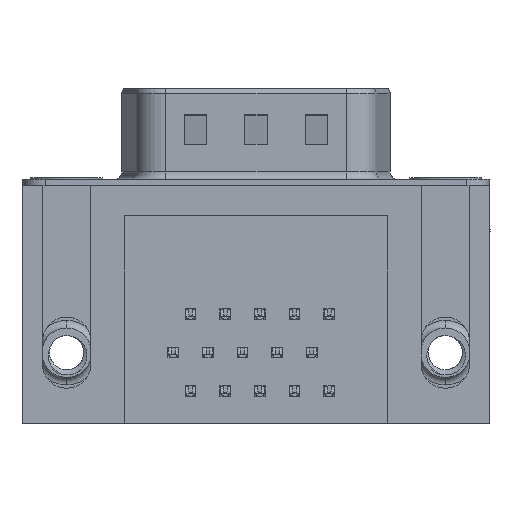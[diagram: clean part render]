
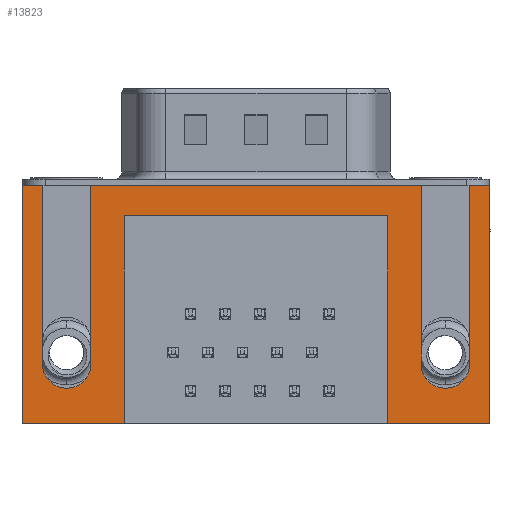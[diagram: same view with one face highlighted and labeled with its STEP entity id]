
A CAD part, front view. The second image highlights one B-rep face of the part: STEP entity #13823.
In plain terms, the highlighted planar face has unit normal (0, -1, 0).
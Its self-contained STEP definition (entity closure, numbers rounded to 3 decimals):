
#106 = DIRECTION ( 'NONE',  ( 0., 0., 1. ) ) ;
#407 = DIRECTION ( 'NONE',  ( 0., -1., 0. ) ) ;
#467 = ORIENTED_EDGE ( 'NONE', *, *, #11216, .F. ) ;
#515 = DIRECTION ( 'NONE',  ( 1., 0., 0. ) ) ;
#764 = VERTEX_POINT ( 'NONE', #19574 ) ;
#930 = CARTESIAN_POINT ( 'NONE',  ( -1.6, -6.275, 0. ) ) ;
#1017 = CARTESIAN_POINT ( 'NONE',  ( 26.59, -6.275, 0. ) ) ;
#1117 = CARTESIAN_POINT ( 'NONE',  ( -2.91, -6.275, -2.5 ) ) ;
#1310 = CARTESIAN_POINT ( 'NONE',  ( 23.39, -6.275, -11.78 ) ) ;
#1505 = EDGE_CURVE ( 'NONE', #8039, #16333, #14740, .T. ) ;
#1553 = VECTOR ( 'NONE', #17499, 1000. ) ;
#1867 = AXIS2_PLACEMENT_3D ( 'NONE', #20007, #10020, #106 ) ;
#1883 = LINE ( 'NONE', #6832, #10170 ) ;
#1933 = EDGE_CURVE ( 'NONE', #10922, #8039, #16270, .T. ) ;
#2094 = CARTESIAN_POINT ( 'NONE',  ( 26.59, -6.275, 0. ) ) ;
#2270 = ORIENTED_EDGE ( 'NONE', *, *, #19438, .F. ) ;
#2291 = DIRECTION ( 'NONE',  ( 0., 0., 1. ) ) ;
#2579 = VECTOR ( 'NONE', #10424, 1000. ) ;
#2657 = DIRECTION ( 'NONE',  ( 0., 0., -1. ) ) ;
#2797 = ORIENTED_EDGE ( 'NONE', *, *, #4100, .F. ) ;
#2808 = FACE_OUTER_BOUND ( 'NONE', #17017, .T. ) ;
#2905 = CARTESIAN_POINT ( 'NONE',  ( 27.9, -6.275, -2.5 ) ) ;
#2934 = VERTEX_POINT ( 'NONE', #20916 ) ;
#3137 = LINE ( 'NONE', #3846, #11400 ) ;
#3655 = LINE ( 'NONE', #18631, #11928 ) ;
#3657 = DIRECTION ( 'NONE',  ( 0., 0., 1. ) ) ;
#3846 = CARTESIAN_POINT ( 'NONE',  ( -2.91, -6.275, 0. ) ) ;
#3973 = CARTESIAN_POINT ( 'NONE',  ( 3.79, -6.275, -2. ) ) ;
#4032 = EDGE_CURVE ( 'NONE', #13349, #19043, #15791, .T. ) ;
#4100 = EDGE_CURVE ( 'NONE', #18681, #9261, #14753, .T. ) ;
#4137 = DIRECTION ( 'NONE',  ( -1., 0., 0. ) ) ;
#4527 = CARTESIAN_POINT ( 'NONE',  ( 23.39, -6.275, 0. ) ) ;
#4547 = EDGE_CURVE ( 'NONE', #9043, #7284, #19715, .T. ) ;
#4594 = CARTESIAN_POINT ( 'NONE',  ( 27.9, -6.275, 0. ) ) ;
#4648 = CARTESIAN_POINT ( 'NONE',  ( 1.6, -6.275, -11.78 ) ) ;
#4765 = VERTEX_POINT ( 'NONE', #12665 ) ;
#4778 = ORIENTED_EDGE ( 'NONE', *, *, #17791, .F. ) ;
#4785 = CARTESIAN_POINT ( 'NONE',  ( 27.9, -6.275, -15.7 ) ) ;
#5122 = CARTESIAN_POINT ( 'NONE',  ( -2.91, -6.275, 0. ) ) ;
#5206 = VECTOR ( 'NONE', #14465, 1000. ) ;
#5345 = VERTEX_POINT ( 'NONE', #4785 ) ;
#5378 = AXIS2_PLACEMENT_3D ( 'NONE', #10319, #407, #11957 ) ;
#5626 = ORIENTED_EDGE ( 'NONE', *, *, #19762, .F. ) ;
#5706 = AXIS2_PLACEMENT_3D ( 'NONE', #1117, #17706, #7795 ) ;
#5830 = CARTESIAN_POINT ( 'NONE',  ( 3.79, -6.275, -2. ) ) ;
#5968 = VECTOR ( 'NONE', #15062, 1000. ) ;
#6076 = CARTESIAN_POINT ( 'NONE',  ( 21.2, -6.275, -2. ) ) ;
#6199 = DIRECTION ( 'NONE',  ( 0., 0., -1. ) ) ;
#6203 = EDGE_CURVE ( 'NONE', #7284, #20278, #16646, .T. ) ;
#6571 = VECTOR ( 'NONE', #2657, 1000. ) ;
#6599 = DIRECTION ( 'NONE',  ( 0., 0., -1. ) ) ;
#6826 = DIRECTION ( 'NONE',  ( 1., 0., 0. ) ) ;
#6832 = CARTESIAN_POINT ( 'NONE',  ( -2.91, -6.275, 0. ) ) ;
#7178 = CARTESIAN_POINT ( 'NONE',  ( -2.91, -6.275, -2.5 ) ) ;
#7284 = VERTEX_POINT ( 'NONE', #6076 ) ;
#7589 = VECTOR ( 'NONE', #6826, 1000. ) ;
#7609 = CARTESIAN_POINT ( 'NONE',  ( 27.9, -6.275, -15.7 ) ) ;
#7769 = ORIENTED_EDGE ( 'NONE', *, *, #4032, .F. ) ;
#7795 = DIRECTION ( 'NONE',  ( 0., 0., -1. ) ) ;
#7887 = CARTESIAN_POINT ( 'NONE',  ( -1.6, -6.275, 0. ) ) ;
#8039 = VERTEX_POINT ( 'NONE', #4648 ) ;
#8467 = DIRECTION ( 'NONE',  ( 1., 0., 0. ) ) ;
#8896 = ORIENTED_EDGE ( 'NONE', *, *, #4547, .F. ) ;
#9043 = VERTEX_POINT ( 'NONE', #17432 ) ;
#9144 = AXIS2_PLACEMENT_3D ( 'NONE', #12203, #15199, #14990 ) ;
#9261 = VERTEX_POINT ( 'NONE', #17936 ) ;
#9319 = ORIENTED_EDGE ( 'NONE', *, *, #20046, .F. ) ;
#9422 = CARTESIAN_POINT ( 'NONE',  ( 0., -6.275, -11.78 ) ) ;
#9679 = EDGE_CURVE ( 'NONE', #4765, #12709, #16786, .T. ) ;
#9837 = CARTESIAN_POINT ( 'NONE',  ( 1.6, -6.275, 0. ) ) ;
#10020 = DIRECTION ( 'NONE',  ( 0., -1., 0. ) ) ;
#10170 = VECTOR ( 'NONE', #8467, 1000. ) ;
#10319 = CARTESIAN_POINT ( 'NONE',  ( 24.99, -6.275, -11.78 ) ) ;
#10338 = LINE ( 'NONE', #7178, #18117 ) ;
#10424 = DIRECTION ( 'NONE',  ( 0., 0., 1. ) ) ;
#10907 = VERTEX_POINT ( 'NONE', #7887 ) ;
#10922 = VERTEX_POINT ( 'NONE', #19573 ) ;
#10967 = AXIS2_PLACEMENT_3D ( 'NONE', #9422, #21039, #11031 ) ;
#11015 = PLANE ( 'NONE',  #5706 ) ;
#11031 = DIRECTION ( 'NONE',  ( 0., 0., -1. ) ) ;
#11216 = EDGE_CURVE ( 'NONE', #12709, #764, #15678, .T. ) ;
#11400 = VECTOR ( 'NONE', #515, 1000. ) ;
#11739 = CARTESIAN_POINT ( 'NONE',  ( 3.79, -6.275, -15.7 ) ) ;
#11928 = VECTOR ( 'NONE', #20352, 1000. ) ;
#11957 = DIRECTION ( 'NONE',  ( 0., 0., 1. ) ) ;
#12162 = CIRCLE ( 'NONE', #10967, 1.6 ) ;
#12203 = CARTESIAN_POINT ( 'NONE',  ( 0., -6.275, -11.78 ) ) ;
#12208 = VECTOR ( 'NONE', #4137, 1000. ) ;
#12433 = VECTOR ( 'NONE', #6599, 1000. ) ;
#12665 = CARTESIAN_POINT ( 'NONE',  ( 23.39, -6.275, 0. ) ) ;
#12709 = VERTEX_POINT ( 'NONE', #1310 ) ;
#13349 = VERTEX_POINT ( 'NONE', #14742 ) ;
#13560 = CARTESIAN_POINT ( 'NONE',  ( 21.2, -6.275, -2. ) ) ;
#13649 = EDGE_CURVE ( 'NONE', #9261, #2934, #10338, .T. ) ;
#13823 = ADVANCED_FACE ( 'NONE', ( #2808 ), #11015, .T. ) ;
#14294 = LINE ( 'NONE', #930, #6571 ) ;
#14465 = DIRECTION ( 'NONE',  ( 0., 0., 1. ) ) ;
#14740 = LINE ( 'NONE', #18696, #5968 ) ;
#14742 = CARTESIAN_POINT ( 'NONE',  ( 26.59, -6.275, -11.78 ) ) ;
#14753 = LINE ( 'NONE', #7609, #1553 ) ;
#14880 = VERTEX_POINT ( 'NONE', #17090 ) ;
#14990 = DIRECTION ( 'NONE',  ( 0., 0., -1. ) ) ;
#15062 = DIRECTION ( 'NONE',  ( 0., 0., 1. ) ) ;
#15199 = DIRECTION ( 'NONE',  ( 0., -1., 0. ) ) ;
#15264 = VECTOR ( 'NONE', #3657, 1000. ) ;
#15678 = CIRCLE ( 'NONE', #5378, 1.6 ) ;
#15791 = LINE ( 'NONE', #2094, #2579 ) ;
#15833 = ORIENTED_EDGE ( 'NONE', *, *, #19524, .F. ) ;
#15864 = ORIENTED_EDGE ( 'NONE', *, *, #21182, .F. ) ;
#16270 = CIRCLE ( 'NONE', #9144, 1.6 ) ;
#16333 = VERTEX_POINT ( 'NONE', #9837 ) ;
#16646 = LINE ( 'NONE', #5830, #12208 ) ;
#16786 = LINE ( 'NONE', #4527, #20736 ) ;
#16881 = LINE ( 'NONE', #21528, #12433 ) ;
#16993 = ORIENTED_EDGE ( 'NONE', *, *, #1505, .F. ) ;
#17017 = EDGE_LOOP ( 'NONE', ( #7769, #15864, #467, #19825, #20773, #16993, #19281, #5626, #4778, #15833, #17101, #2797, #19601, #17861, #8896, #2270, #21110, #9319 ) ) ;
#17090 = CARTESIAN_POINT ( 'NONE',  ( -1.6, -6.275, -11.78 ) ) ;
#17101 = ORIENTED_EDGE ( 'NONE', *, *, #13649, .F. ) ;
#17432 = CARTESIAN_POINT ( 'NONE',  ( 21.2, -6.275, -15.7 ) ) ;
#17499 = DIRECTION ( 'NONE',  ( -1., 0., 0. ) ) ;
#17706 = DIRECTION ( 'NONE',  ( 0., -1., 0. ) ) ;
#17791 = EDGE_CURVE ( 'NONE', #10907, #14880, #14294, .T. ) ;
#17861 = ORIENTED_EDGE ( 'NONE', *, *, #6203, .F. ) ;
#17899 = LINE ( 'NONE', #2905, #5206 ) ;
#17936 = CARTESIAN_POINT ( 'NONE',  ( -2.91, -6.275, -15.7 ) ) ;
#18009 = EDGE_CURVE ( 'NONE', #16333, #4765, #1883, .T. ) ;
#18117 = VECTOR ( 'NONE', #2291, 1000. ) ;
#18152 = CIRCLE ( 'NONE', #1867, 1.6 ) ;
#18631 = CARTESIAN_POINT ( 'NONE',  ( 27.9, -6.275, -15.7 ) ) ;
#18681 = VERTEX_POINT ( 'NONE', #11739 ) ;
#18696 = CARTESIAN_POINT ( 'NONE',  ( 1.6, -6.275, 0. ) ) ;
#19043 = VERTEX_POINT ( 'NONE', #1017 ) ;
#19115 = EDGE_CURVE ( 'NONE', #5345, #21005, #17899, .T. ) ;
#19281 = ORIENTED_EDGE ( 'NONE', *, *, #1933, .F. ) ;
#19438 = EDGE_CURVE ( 'NONE', #5345, #9043, #3655, .T. ) ;
#19524 = EDGE_CURVE ( 'NONE', #2934, #10907, #3137, .T. ) ;
#19573 = CARTESIAN_POINT ( 'NONE',  ( 0., -6.275, -13.38 ) ) ;
#19574 = CARTESIAN_POINT ( 'NONE',  ( 24.99, -6.275, -13.38 ) ) ;
#19601 = ORIENTED_EDGE ( 'NONE', *, *, #20531, .F. ) ;
#19715 = LINE ( 'NONE', #13560, #15264 ) ;
#19762 = EDGE_CURVE ( 'NONE', #14880, #10922, #12162, .T. ) ;
#19825 = ORIENTED_EDGE ( 'NONE', *, *, #9679, .F. ) ;
#20007 = CARTESIAN_POINT ( 'NONE',  ( 24.99, -6.275, -11.78 ) ) ;
#20046 = EDGE_CURVE ( 'NONE', #19043, #21005, #20846, .T. ) ;
#20278 = VERTEX_POINT ( 'NONE', #3973 ) ;
#20352 = DIRECTION ( 'NONE',  ( -1., 0., 0. ) ) ;
#20531 = EDGE_CURVE ( 'NONE', #20278, #18681, #16881, .T. ) ;
#20736 = VECTOR ( 'NONE', #6199, 1000. ) ;
#20773 = ORIENTED_EDGE ( 'NONE', *, *, #18009, .F. ) ;
#20846 = LINE ( 'NONE', #5122, #7589 ) ;
#20916 = CARTESIAN_POINT ( 'NONE',  ( -2.91, -6.275, 0. ) ) ;
#21005 = VERTEX_POINT ( 'NONE', #4594 ) ;
#21039 = DIRECTION ( 'NONE',  ( 0., -1., 0. ) ) ;
#21110 = ORIENTED_EDGE ( 'NONE', *, *, #19115, .T. ) ;
#21182 = EDGE_CURVE ( 'NONE', #764, #13349, #18152, .T. ) ;
#21528 = CARTESIAN_POINT ( 'NONE',  ( 3.79, -6.275, -2. ) ) ;
